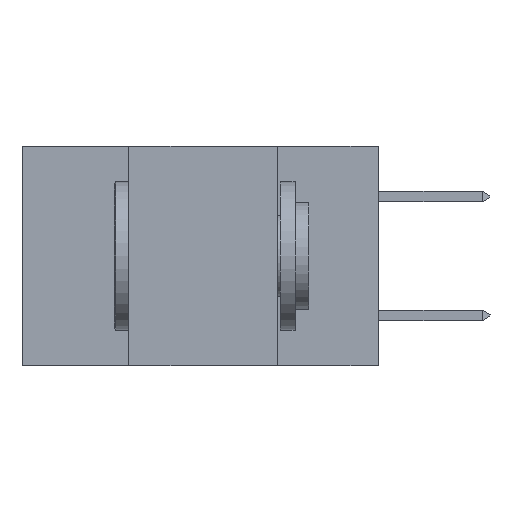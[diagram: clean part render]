
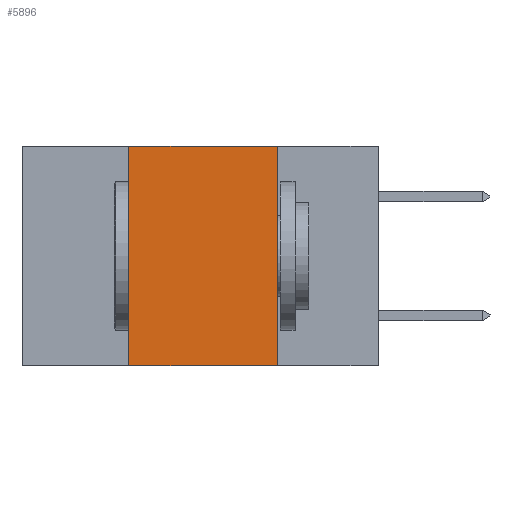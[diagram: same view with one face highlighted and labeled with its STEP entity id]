
A CAD part, left-side view. The second image highlights one B-rep face of the part: STEP entity #5896.
In plain terms, the highlighted planar face has unit normal (-1, 0, 0).
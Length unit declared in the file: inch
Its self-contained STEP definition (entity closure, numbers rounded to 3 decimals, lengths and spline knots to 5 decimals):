
#100 = LINE ( 'NONE', #7033, #12075 ) ;
#277 = CARTESIAN_POINT ( 'NONE',  ( 0., 0.6, 0. ) ) ;
#405 = DIRECTION ( 'NONE',  ( 0., -1., 0. ) ) ;
#417 = VECTOR ( 'NONE', #2453, 39.37008 ) ;
#2453 = DIRECTION ( 'NONE',  ( 0., -1., 0. ) ) ;
#2580 = EDGE_CURVE ( 'NONE', #10406, #8801, #13684, .T. ) ;
#2838 = CARTESIAN_POINT ( 'NONE',  ( 0., 0.42, -0.37 ) ) ;
#4278 = FACE_OUTER_BOUND ( 'NONE', #6771, .T. ) ;
#4397 = VERTEX_POINT ( 'NONE', #6634 ) ;
#4547 = ORIENTED_EDGE ( 'NONE', *, *, #9088, .F. ) ;
#4669 = CARTESIAN_POINT ( 'NONE',  ( 0., 0.42, 0. ) ) ;
#5809 = DIRECTION ( 'NONE',  ( 0., 0., -1. ) ) ;
#5896 = ADVANCED_FACE ( 'NONE', ( #4278 ), #12159, .F. ) ;
#6634 = CARTESIAN_POINT ( 'NONE',  ( 0., 0.42, 0. ) ) ;
#6771 = EDGE_LOOP ( 'NONE', ( #4547, #7475, #12603, #8528 ) ) ;
#6786 = CARTESIAN_POINT ( 'NONE',  ( 0., 0.6, 0. ) ) ;
#7012 = CARTESIAN_POINT ( 'NONE',  ( 0., 0.17, 0. ) ) ;
#7033 = CARTESIAN_POINT ( 'NONE',  ( 0., 0.17, 0. ) ) ;
#7475 = ORIENTED_EDGE ( 'NONE', *, *, #10797, .F. ) ;
#7491 = VECTOR ( 'NONE', #12195, 39.37008 ) ;
#7563 = CARTESIAN_POINT ( 'NONE',  ( 0., 0.17, -0.37 ) ) ;
#7902 = DIRECTION ( 'NONE',  ( 1., 0., 0. ) ) ;
#8275 = EDGE_CURVE ( 'NONE', #10406, #4397, #9701, .T. ) ;
#8528 = ORIENTED_EDGE ( 'NONE', *, *, #2580, .T. ) ;
#8801 = VERTEX_POINT ( 'NONE', #7563 ) ;
#8958 = VECTOR ( 'NONE', #405, 39.37008 ) ;
#9088 = EDGE_CURVE ( 'NONE', #12920, #8801, #100, .T. ) ;
#9156 = CARTESIAN_POINT ( 'NONE',  ( 0., 0.6, -0.37 ) ) ;
#9701 = LINE ( 'NONE', #4669, #7491 ) ;
#10406 = VERTEX_POINT ( 'NONE', #2838 ) ;
#10797 = EDGE_CURVE ( 'NONE', #4397, #12920, #12370, .T. ) ;
#11178 = DIRECTION ( 'NONE',  ( 0., 0., -1. ) ) ;
#12075 = VECTOR ( 'NONE', #5809, 39.37008 ) ;
#12159 = PLANE ( 'NONE',  #12757 ) ;
#12195 = DIRECTION ( 'NONE',  ( 0., 0., 1. ) ) ;
#12370 = LINE ( 'NONE', #277, #417 ) ;
#12603 = ORIENTED_EDGE ( 'NONE', *, *, #8275, .F. ) ;
#12757 = AXIS2_PLACEMENT_3D ( 'NONE', #6786, #7902, #11178 ) ;
#12920 = VERTEX_POINT ( 'NONE', #7012 ) ;
#13684 = LINE ( 'NONE', #9156, #8958 ) ;
